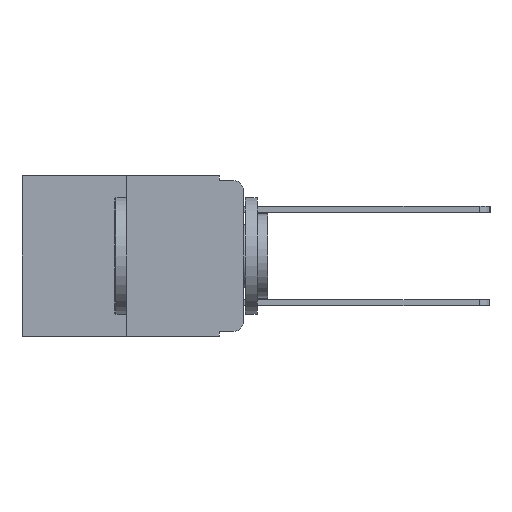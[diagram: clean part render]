
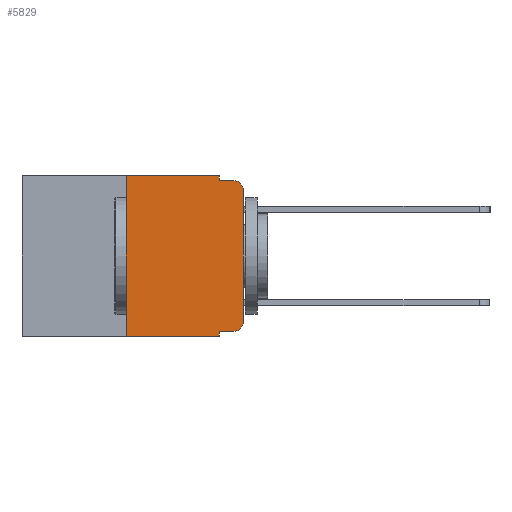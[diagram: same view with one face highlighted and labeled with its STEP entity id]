
A CAD part, left-side view. The second image highlights one B-rep face of the part: STEP entity #5829.
In plain terms, the highlighted planar face has unit normal (-1, 0, 0).
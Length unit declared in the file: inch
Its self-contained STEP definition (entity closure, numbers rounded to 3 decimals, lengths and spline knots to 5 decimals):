
#29 = LINE ( 'NONE', #5565, #9292 ) ;
#52 = CARTESIAN_POINT ( 'NONE',  ( 0., 0.473, 0. ) ) ;
#95 = CARTESIAN_POINT ( 'NONE',  ( 0., 0., -0.313 ) ) ;
#248 = CARTESIAN_POINT ( 'NONE',  ( 0., 0.02, -0.333 ) ) ;
#441 = ORIENTED_EDGE ( 'NONE', *, *, #12403, .T. ) ;
#854 = VERTEX_POINT ( 'NONE', #248 ) ;
#886 = ORIENTED_EDGE ( 'NONE', *, *, #1656, .F. ) ;
#1111 = DIRECTION ( 'NONE',  ( 0., 0., -1. ) ) ;
#1126 = VECTOR ( 'NONE', #7229, 39.37008 ) ;
#1272 = VERTEX_POINT ( 'NONE', #3651 ) ;
#1656 = EDGE_CURVE ( 'NONE', #1272, #6614, #7124, .T. ) ;
#1960 = DIRECTION ( 'NONE',  ( 0., 0., -1. ) ) ;
#2215 = CARTESIAN_POINT ( 'NONE',  ( 0., 0.02, -0.03 ) ) ;
#2381 = AXIS2_PLACEMENT_3D ( 'NONE', #3712, #11586, #4861 ) ;
#2548 = VERTEX_POINT ( 'NONE', #7565 ) ;
#2607 = VECTOR ( 'NONE', #10422, 39.37008 ) ;
#2791 = DIRECTION ( 'NONE',  ( 0., -1., 0. ) ) ;
#2980 = VECTOR ( 'NONE', #1111, 39.37008 ) ;
#3257 = CIRCLE ( 'NONE', #2381, 0.02 ) ;
#3457 = DIRECTION ( 'NONE',  ( 0., 0., -1. ) ) ;
#3556 = ORIENTED_EDGE ( 'NONE', *, *, #13115, .T. ) ;
#3651 = CARTESIAN_POINT ( 'NONE',  ( 0., 0.25, 0. ) ) ;
#3712 = CARTESIAN_POINT ( 'NONE',  ( 0., 0.02, -0.313 ) ) ;
#3876 = VERTEX_POINT ( 'NONE', #14529 ) ;
#4035 = DIRECTION ( 'NONE',  ( 1., 0., 0. ) ) ;
#4128 = VERTEX_POINT ( 'NONE', #13807 ) ;
#4398 = CARTESIAN_POINT ( 'NONE',  ( 0., 0.051, -0.333 ) ) ;
#4558 = VERTEX_POINT ( 'NONE', #9977 ) ;
#4660 = ORIENTED_EDGE ( 'NONE', *, *, #14286, .T. ) ;
#4753 = CARTESIAN_POINT ( 'NONE',  ( 0., 0.051, -0.01 ) ) ;
#4861 = DIRECTION ( 'NONE',  ( 0., 0., -1. ) ) ;
#4972 = CARTESIAN_POINT ( 'NONE',  ( 0., 0.25, -0.343 ) ) ;
#4998 = ORIENTED_EDGE ( 'NONE', *, *, #7978, .T. ) ;
#5221 = LINE ( 'NONE', #4398, #11205 ) ;
#5565 = CARTESIAN_POINT ( 'NONE',  ( 0., 0.051, 0. ) ) ;
#5707 = LINE ( 'NONE', #4753, #2607 ) ;
#5742 = AXIS2_PLACEMENT_3D ( 'NONE', #2215, #10263, #3457 ) ;
#5829 = ADVANCED_FACE ( 'NONE', ( #8610 ), #9671, .F. ) ;
#5855 = LINE ( 'NONE', #12529, #6214 ) ;
#6050 = CARTESIAN_POINT ( 'NONE',  ( 0., 0.25, 0. ) ) ;
#6214 = VECTOR ( 'NONE', #8160, 39.37008 ) ;
#6296 = CARTESIAN_POINT ( 'NONE',  ( 0., 0.473, 0. ) ) ;
#6614 = VERTEX_POINT ( 'NONE', #10902 ) ;
#6750 = DIRECTION ( 'NONE',  ( 0., -1., 0. ) ) ;
#7004 = ORIENTED_EDGE ( 'NONE', *, *, #11679, .F. ) ;
#7124 = LINE ( 'NONE', #6296, #9715 ) ;
#7158 = CARTESIAN_POINT ( 'NONE',  ( 0., 0.051, 0. ) ) ;
#7215 = VERTEX_POINT ( 'NONE', #4972 ) ;
#7229 = DIRECTION ( 'NONE',  ( 0., 0., 1. ) ) ;
#7270 = AXIS2_PLACEMENT_3D ( 'NONE', #52, #4035, #11883 ) ;
#7539 = LINE ( 'NONE', #6050, #1126 ) ;
#7565 = CARTESIAN_POINT ( 'NONE',  ( 0., 0.051, -0.343 ) ) ;
#7667 = CIRCLE ( 'NONE', #5742, 0.02 ) ;
#7706 = ORIENTED_EDGE ( 'NONE', *, *, #9471, .F. ) ;
#7978 = EDGE_CURVE ( 'NONE', #854, #9865, #3257, .T. ) ;
#8160 = DIRECTION ( 'NONE',  ( 0., 0., 1. ) ) ;
#8330 = VECTOR ( 'NONE', #2791, 39.37008 ) ;
#8512 = VERTEX_POINT ( 'NONE', #13982 ) ;
#8527 = EDGE_LOOP ( 'NONE', ( #3556, #441, #7004, #12862, #886, #10305, #4660, #7706, #10651, #4998 ) ) ;
#8610 = FACE_OUTER_BOUND ( 'NONE', #8527, .T. ) ;
#8669 = LINE ( 'NONE', #10756, #8330 ) ;
#8704 = EDGE_CURVE ( 'NONE', #4128, #854, #5221, .T. ) ;
#9292 = VECTOR ( 'NONE', #1960, 39.37008 ) ;
#9471 = EDGE_CURVE ( 'NONE', #4128, #2548, #29, .T. ) ;
#9671 = PLANE ( 'NONE',  #7270 ) ;
#9715 = VECTOR ( 'NONE', #6750, 39.37008 ) ;
#9865 = VERTEX_POINT ( 'NONE', #95 ) ;
#9977 = CARTESIAN_POINT ( 'NONE',  ( 0., 0., -0.03 ) ) ;
#10217 = EDGE_CURVE ( 'NONE', #7215, #1272, #7539, .T. ) ;
#10263 = DIRECTION ( 'NONE',  ( -1., 0., 0. ) ) ;
#10305 = ORIENTED_EDGE ( 'NONE', *, *, #10217, .F. ) ;
#10422 = DIRECTION ( 'NONE',  ( 0., -1., 0. ) ) ;
#10651 = ORIENTED_EDGE ( 'NONE', *, *, #8704, .T. ) ;
#10756 = CARTESIAN_POINT ( 'NONE',  ( 0., 0.473, -0.343 ) ) ;
#10902 = CARTESIAN_POINT ( 'NONE',  ( 0., 0.051, 0. ) ) ;
#10953 = EDGE_CURVE ( 'NONE', #6614, #3876, #14847, .T. ) ;
#11205 = VECTOR ( 'NONE', #12223, 39.37008 ) ;
#11586 = DIRECTION ( 'NONE',  ( -1., 0., 0. ) ) ;
#11679 = EDGE_CURVE ( 'NONE', #3876, #8512, #5707, .T. ) ;
#11883 = DIRECTION ( 'NONE',  ( 0., 0., -1. ) ) ;
#12223 = DIRECTION ( 'NONE',  ( 0., -1., 0. ) ) ;
#12403 = EDGE_CURVE ( 'NONE', #4558, #8512, #7667, .T. ) ;
#12529 = CARTESIAN_POINT ( 'NONE',  ( 0., 0., 0. ) ) ;
#12862 = ORIENTED_EDGE ( 'NONE', *, *, #10953, .F. ) ;
#13115 = EDGE_CURVE ( 'NONE', #9865, #4558, #5855, .T. ) ;
#13807 = CARTESIAN_POINT ( 'NONE',  ( 0., 0.051, -0.333 ) ) ;
#13982 = CARTESIAN_POINT ( 'NONE',  ( 0., 0.02, -0.01 ) ) ;
#14286 = EDGE_CURVE ( 'NONE', #7215, #2548, #8669, .T. ) ;
#14529 = CARTESIAN_POINT ( 'NONE',  ( 0., 0.051, -0.01 ) ) ;
#14847 = LINE ( 'NONE', #7158, #2980 ) ;
